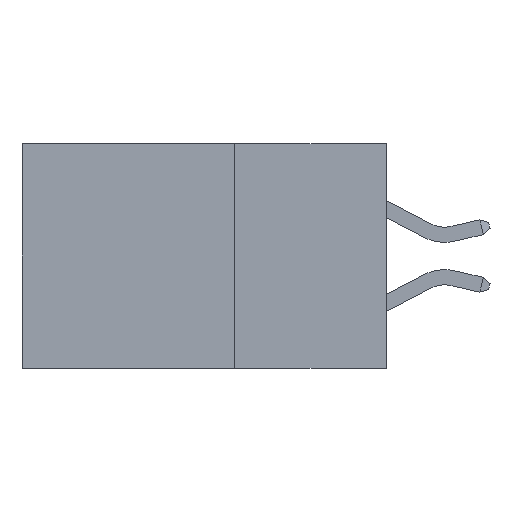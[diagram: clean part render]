
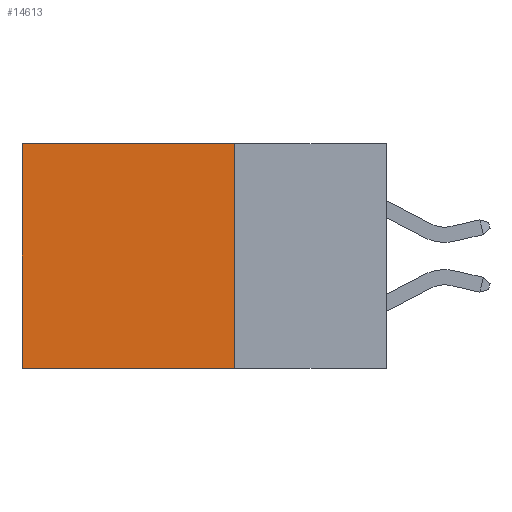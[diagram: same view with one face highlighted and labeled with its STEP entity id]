
A CAD part, left-side view. The second image highlights one B-rep face of the part: STEP entity #14613.
In plain terms, the highlighted planar face has unit normal (-1, 0, 0).
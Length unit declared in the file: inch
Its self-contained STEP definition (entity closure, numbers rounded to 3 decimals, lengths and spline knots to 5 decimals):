
#526 = CARTESIAN_POINT ( 'NONE',  ( 0.298, 0.6, -0.37 ) ) ;
#547 = VECTOR ( 'NONE', #14076, 39.37008 ) ;
#1622 = ORIENTED_EDGE ( 'NONE', *, *, #5520, .F. ) ;
#1787 = CARTESIAN_POINT ( 'NONE',  ( 0.298, 0.25, 0. ) ) ;
#1807 = CARTESIAN_POINT ( 'NONE',  ( 0.298, 0.25, -0.37 ) ) ;
#1931 = VERTEX_POINT ( 'NONE', #6794 ) ;
#2445 = DIRECTION ( 'NONE',  ( 1., 0., 0. ) ) ;
#2546 = VECTOR ( 'NONE', #9745, 39.37008 ) ;
#2622 = LINE ( 'NONE', #1807, #14075 ) ;
#2658 = DIRECTION ( 'NONE',  ( 0., 0., -1. ) ) ;
#3408 = DIRECTION ( 'NONE',  ( 0., 0., -1. ) ) ;
#3589 = VERTEX_POINT ( 'NONE', #526 ) ;
#4108 = CARTESIAN_POINT ( 'NONE',  ( 0.298, 0.25, 0. ) ) ;
#4579 = LINE ( 'NONE', #7102, #7574 ) ;
#5364 = LINE ( 'NONE', #4108, #547 ) ;
#5520 = EDGE_CURVE ( 'NONE', #5622, #3589, #2622, .T. ) ;
#5622 = VERTEX_POINT ( 'NONE', #6966 ) ;
#6794 = CARTESIAN_POINT ( 'NONE',  ( 0.298, 0.25, 0. ) ) ;
#6966 = CARTESIAN_POINT ( 'NONE',  ( 0.298, 0.25, -0.37 ) ) ;
#7102 = CARTESIAN_POINT ( 'NONE',  ( 0.298, 0.6, 0. ) ) ;
#7574 = VECTOR ( 'NONE', #2658, 39.37008 ) ;
#8042 = AXIS2_PLACEMENT_3D ( 'NONE', #11275, #2445, #3408 ) ;
#8186 = FACE_OUTER_BOUND ( 'NONE', #12955, .T. ) ;
#8278 = ORIENTED_EDGE ( 'NONE', *, *, #12070, .T. ) ;
#9745 = DIRECTION ( 'NONE',  ( 0., 0., -1. ) ) ;
#9821 = EDGE_CURVE ( 'NONE', #1931, #11930, #5364, .T. ) ;
#10637 = ORIENTED_EDGE ( 'NONE', *, *, #14094, .F. ) ;
#11275 = CARTESIAN_POINT ( 'NONE',  ( 0.298, 0.25, 0. ) ) ;
#11371 = PLANE ( 'NONE',  #8042 ) ;
#11695 = CARTESIAN_POINT ( 'NONE',  ( 0.298, 0.6, 0. ) ) ;
#11923 = DIRECTION ( 'NONE',  ( 0., 1., 0. ) ) ;
#11930 = VERTEX_POINT ( 'NONE', #11695 ) ;
#12070 = EDGE_CURVE ( 'NONE', #11930, #3589, #4579, .T. ) ;
#12955 = EDGE_LOOP ( 'NONE', ( #8278, #1622, #10637, #12966 ) ) ;
#12966 = ORIENTED_EDGE ( 'NONE', *, *, #9821, .T. ) ;
#13491 = LINE ( 'NONE', #1787, #2546 ) ;
#14075 = VECTOR ( 'NONE', #11923, 39.37008 ) ;
#14076 = DIRECTION ( 'NONE',  ( 0., 1., 0. ) ) ;
#14094 = EDGE_CURVE ( 'NONE', #1931, #5622, #13491, .T. ) ;
#14613 = ADVANCED_FACE ( 'NONE', ( #8186 ), #11371, .F. ) ;
